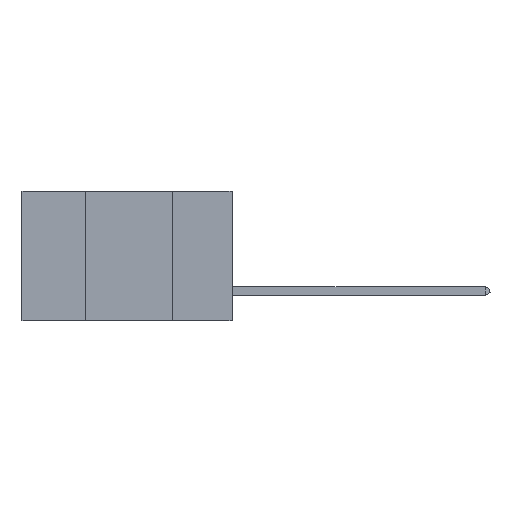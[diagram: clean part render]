
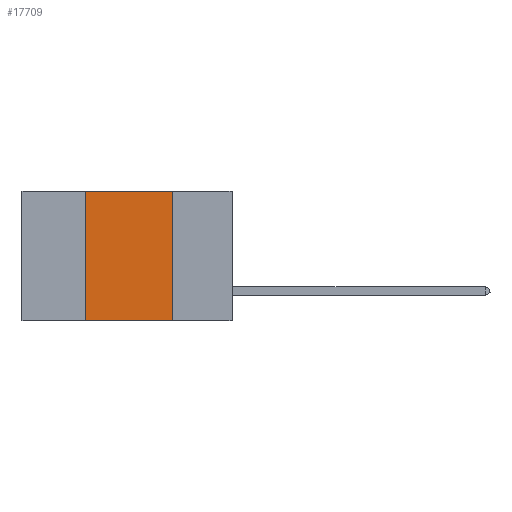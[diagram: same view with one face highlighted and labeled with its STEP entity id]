
A CAD part, left-side view. The second image highlights one B-rep face of the part: STEP entity #17709.
In plain terms, the highlighted planar face has unit normal (-1, 0, 0).
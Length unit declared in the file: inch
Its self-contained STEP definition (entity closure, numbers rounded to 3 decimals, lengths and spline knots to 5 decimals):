
#1130 = DIRECTION ( 'NONE',  ( 0., -1., 0. ) ) ;
#1302 = ORIENTED_EDGE ( 'NONE', *, *, #20852, .T. ) ;
#1334 = CARTESIAN_POINT ( 'NONE',  ( 0., 0.42, -0.37 ) ) ;
#1362 = CARTESIAN_POINT ( 'NONE',  ( 0., 0.6, -0.37 ) ) ;
#1562 = VERTEX_POINT ( 'NONE', #8325 ) ;
#1626 = DIRECTION ( 'NONE',  ( 1., 0., 0. ) ) ;
#1669 = PLANE ( 'NONE',  #3602 ) ;
#2503 = CARTESIAN_POINT ( 'NONE',  ( 0., 0.17, -0.37 ) ) ;
#2668 = LINE ( 'NONE', #14412, #13312 ) ;
#3602 = AXIS2_PLACEMENT_3D ( 'NONE', #5129, #1626, #5894 ) ;
#5129 = CARTESIAN_POINT ( 'NONE',  ( 0., 0.6, 0. ) ) ;
#5894 = DIRECTION ( 'NONE',  ( 0., 0., -1. ) ) ;
#6144 = VECTOR ( 'NONE', #14401, 39.37008 ) ;
#6256 = EDGE_LOOP ( 'NONE', ( #15969, #12211, #15365, #1302 ) ) ;
#7469 = CARTESIAN_POINT ( 'NONE',  ( 0., 0.42, 0. ) ) ;
#7897 = EDGE_CURVE ( 'NONE', #21170, #17745, #19112, .T. ) ;
#8325 = CARTESIAN_POINT ( 'NONE',  ( 0., 0.17, 0. ) ) ;
#9013 = VECTOR ( 'NONE', #17687, 39.37008 ) ;
#9493 = DIRECTION ( 'NONE',  ( 0., -1., 0. ) ) ;
#11754 = VERTEX_POINT ( 'NONE', #2503 ) ;
#12211 = ORIENTED_EDGE ( 'NONE', *, *, #21081, .F. ) ;
#13312 = VECTOR ( 'NONE', #9493, 39.37008 ) ;
#14401 = DIRECTION ( 'NONE',  ( 0., 0., 1. ) ) ;
#14412 = CARTESIAN_POINT ( 'NONE',  ( 0., 0.6, 0. ) ) ;
#15365 = ORIENTED_EDGE ( 'NONE', *, *, #7897, .F. ) ;
#15969 = ORIENTED_EDGE ( 'NONE', *, *, #19401, .F. ) ;
#16227 = LINE ( 'NONE', #17572, #9013 ) ;
#16449 = LINE ( 'NONE', #1362, #21521 ) ;
#17572 = CARTESIAN_POINT ( 'NONE',  ( 0., 0.17, 0. ) ) ;
#17687 = DIRECTION ( 'NONE',  ( 0., 0., -1. ) ) ;
#17709 = ADVANCED_FACE ( 'NONE', ( #22023 ), #1669, .F. ) ;
#17745 = VERTEX_POINT ( 'NONE', #19318 ) ;
#19112 = LINE ( 'NONE', #7469, #6144 ) ;
#19318 = CARTESIAN_POINT ( 'NONE',  ( 0., 0.42, 0. ) ) ;
#19401 = EDGE_CURVE ( 'NONE', #1562, #11754, #16227, .T. ) ;
#20852 = EDGE_CURVE ( 'NONE', #21170, #11754, #16449, .T. ) ;
#21081 = EDGE_CURVE ( 'NONE', #17745, #1562, #2668, .T. ) ;
#21170 = VERTEX_POINT ( 'NONE', #1334 ) ;
#21521 = VECTOR ( 'NONE', #1130, 39.37008 ) ;
#22023 = FACE_OUTER_BOUND ( 'NONE', #6256, .T. ) ;
